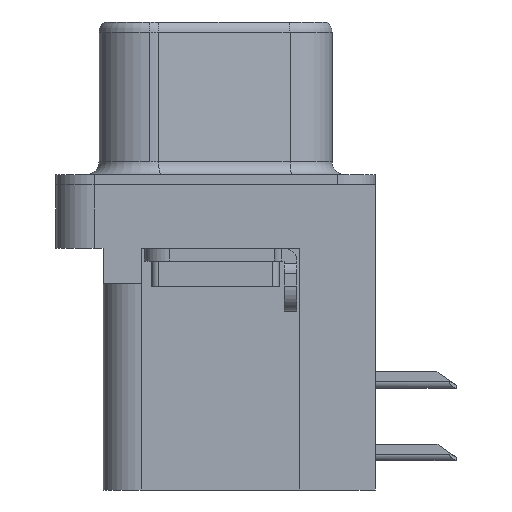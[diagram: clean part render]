
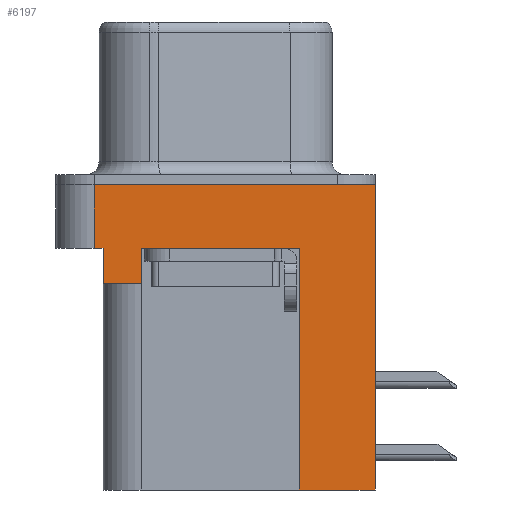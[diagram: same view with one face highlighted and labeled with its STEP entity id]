
A CAD part, left-side view. The second image highlights one B-rep face of the part: STEP entity #6197.
In plain terms, the highlighted planar face has unit normal (-1, 0, 0).
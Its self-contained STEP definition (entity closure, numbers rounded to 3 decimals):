
#368 = VERTEX_POINT ( 'NONE', #7189 ) ;
#403 = DIRECTION ( 'NONE',  ( 0., 0., 1. ) ) ;
#436 = VERTEX_POINT ( 'NONE', #8940 ) ;
#1205 = ORIENTED_EDGE ( 'NONE', *, *, #11665, .F. ) ;
#1232 = DIRECTION ( 'NONE',  ( 0., 1., 0. ) ) ;
#1265 = DIRECTION ( 'NONE',  ( 0., -1., 0. ) ) ;
#1418 = DIRECTION ( 'NONE',  ( 0., 0., 1. ) ) ;
#2307 = DIRECTION ( 'NONE',  ( 0., -1., 0. ) ) ;
#2911 = EDGE_CURVE ( 'NONE', #9592, #368, #12418, .T. ) ;
#3800 = VECTOR ( 'NONE', #9258, 1000. ) ;
#3972 = CARTESIAN_POINT ( 'NONE',  ( -2.91, -3.295, -12. ) ) ;
#4002 = CARTESIAN_POINT ( 'NONE',  ( -2.91, -6.275, -2.5 ) ) ;
#4047 = LINE ( 'NONE', #8004, #3800 ) ;
#4714 = FACE_OUTER_BOUND ( 'NONE', #9419, .T. ) ;
#5123 = CARTESIAN_POINT ( 'NONE',  ( -2.91, -6.275, -2.5 ) ) ;
#5276 = VECTOR ( 'NONE', #5480, 1000. ) ;
#5323 = LINE ( 'NONE', #9266, #5276 ) ;
#5368 = CARTESIAN_POINT ( 'NONE',  ( -2.91, -3.295, -12. ) ) ;
#5480 = DIRECTION ( 'NONE',  ( 0., -1., 0. ) ) ;
#5644 = CARTESIAN_POINT ( 'NONE',  ( -2.91, 2.895, -3.9 ) ) ;
#5787 = EDGE_CURVE ( 'NONE', #368, #7669, #5323, .T. ) ;
#5891 = CARTESIAN_POINT ( 'NONE',  ( -2.91, -6.275, -2.5 ) ) ;
#6053 = AXIS2_PLACEMENT_3D ( 'NONE', #5891, #14298, #7161 ) ;
#6106 = ORIENTED_EDGE ( 'NONE', *, *, #10498, .F. ) ;
#6197 = ADVANCED_FACE ( 'NONE', ( #4714 ), #13156, .T. ) ;
#6311 = VECTOR ( 'NONE', #2307, 1000. ) ;
#6359 = LINE ( 'NONE', #9940, #6311 ) ;
#6363 = CARTESIAN_POINT ( 'NONE',  ( -2.91, 2.895, -3.9 ) ) ;
#7161 = DIRECTION ( 'NONE',  ( 0., 0., 1. ) ) ;
#7189 = CARTESIAN_POINT ( 'NONE',  ( -2.91, 2.895, -2.5 ) ) ;
#7432 = VERTEX_POINT ( 'NONE', #11714 ) ;
#7538 = VECTOR ( 'NONE', #1265, 1000. ) ;
#7648 = LINE ( 'NONE', #4002, #7538 ) ;
#7669 = VERTEX_POINT ( 'NONE', #12248 ) ;
#7828 = DIRECTION ( 'NONE',  ( 0., 0., 1. ) ) ;
#8004 = CARTESIAN_POINT ( 'NONE',  ( -2.91, 4.425, -3.9 ) ) ;
#8096 = VERTEX_POINT ( 'NONE', #12375 ) ;
#8150 = ORIENTED_EDGE ( 'NONE', *, *, #11208, .T. ) ;
#8847 = EDGE_CURVE ( 'NONE', #8096, #12609, #12867, .T. ) ;
#8940 = CARTESIAN_POINT ( 'NONE',  ( -2.91, 4.425, -3.9 ) ) ;
#9080 = VECTOR ( 'NONE', #403, 1000. ) ;
#9115 = LINE ( 'NONE', #9463, #9080 ) ;
#9193 = CARTESIAN_POINT ( 'NONE',  ( -2.91, -3.295, -12. ) ) ;
#9258 = DIRECTION ( 'NONE',  ( 0., 1., 0. ) ) ;
#9266 = CARTESIAN_POINT ( 'NONE',  ( -2.91, -6.275, -2.5 ) ) ;
#9419 = EDGE_LOOP ( 'NONE', ( #1205, #10575, #8150, #6106, #12833, #13046, #10346, #10182, #15277, #14579 ) ) ;
#9463 = CARTESIAN_POINT ( 'NONE',  ( -2.91, 4.425, -3.9 ) ) ;
#9556 = VECTOR ( 'NONE', #7828, 1000. ) ;
#9577 = EDGE_CURVE ( 'NONE', #9665, #7432, #11133, .T. ) ;
#9579 = LINE ( 'NONE', #5368, #9556 ) ;
#9592 = VERTEX_POINT ( 'NONE', #6363 ) ;
#9665 = VERTEX_POINT ( 'NONE', #15819 ) ;
#9672 = EDGE_CURVE ( 'NONE', #9665, #10332, #10805, .T. ) ;
#9940 = CARTESIAN_POINT ( 'NONE',  ( -2.91, -6.275, 0. ) ) ;
#10182 = ORIENTED_EDGE ( 'NONE', *, *, #10314, .F. ) ;
#10314 = EDGE_CURVE ( 'NONE', #10332, #7669, #9579, .T. ) ;
#10332 = VERTEX_POINT ( 'NONE', #9193 ) ;
#10346 = ORIENTED_EDGE ( 'NONE', *, *, #5787, .T. ) ;
#10449 = VERTEX_POINT ( 'NONE', #14063 ) ;
#10498 = EDGE_CURVE ( 'NONE', #436, #10449, #9115, .T. ) ;
#10575 = ORIENTED_EDGE ( 'NONE', *, *, #8847, .F. ) ;
#10784 = VECTOR ( 'NONE', #1232, 1000. ) ;
#10805 = LINE ( 'NONE', #3972, #10784 ) ;
#10995 = VECTOR ( 'NONE', #11282, 1000. ) ;
#11133 = LINE ( 'NONE', #5123, #10995 ) ;
#11208 = EDGE_CURVE ( 'NONE', #8096, #10449, #7648, .T. ) ;
#11282 = DIRECTION ( 'NONE',  ( 0., 0., 1. ) ) ;
#11665 = EDGE_CURVE ( 'NONE', #12609, #7432, #6359, .T. ) ;
#11714 = CARTESIAN_POINT ( 'NONE',  ( -2.91, -6.275, 0. ) ) ;
#12248 = CARTESIAN_POINT ( 'NONE',  ( -2.91, -3.295, -2.5 ) ) ;
#12367 = VECTOR ( 'NONE', #1418, 1000. ) ;
#12375 = CARTESIAN_POINT ( 'NONE',  ( -2.91, 4.775, -2.5 ) ) ;
#12418 = LINE ( 'NONE', #5644, #12367 ) ;
#12608 = EDGE_CURVE ( 'NONE', #9592, #436, #4047, .T. ) ;
#12609 = VERTEX_POINT ( 'NONE', #13917 ) ;
#12760 = VECTOR ( 'NONE', #14384, 1000. ) ;
#12833 = ORIENTED_EDGE ( 'NONE', *, *, #12608, .F. ) ;
#12867 = LINE ( 'NONE', #13255, #12760 ) ;
#13046 = ORIENTED_EDGE ( 'NONE', *, *, #2911, .T. ) ;
#13156 = PLANE ( 'NONE',  #6053 ) ;
#13255 = CARTESIAN_POINT ( 'NONE',  ( -2.91, 4.775, -2.5 ) ) ;
#13917 = CARTESIAN_POINT ( 'NONE',  ( -2.91, 4.775, 0. ) ) ;
#14063 = CARTESIAN_POINT ( 'NONE',  ( -2.91, 4.425, -2.5 ) ) ;
#14298 = DIRECTION ( 'NONE',  ( -1., 0., 0. ) ) ;
#14384 = DIRECTION ( 'NONE',  ( 0., 0., 1. ) ) ;
#14579 = ORIENTED_EDGE ( 'NONE', *, *, #9577, .T. ) ;
#15277 = ORIENTED_EDGE ( 'NONE', *, *, #9672, .F. ) ;
#15819 = CARTESIAN_POINT ( 'NONE',  ( -2.91, -6.275, -12. ) ) ;
